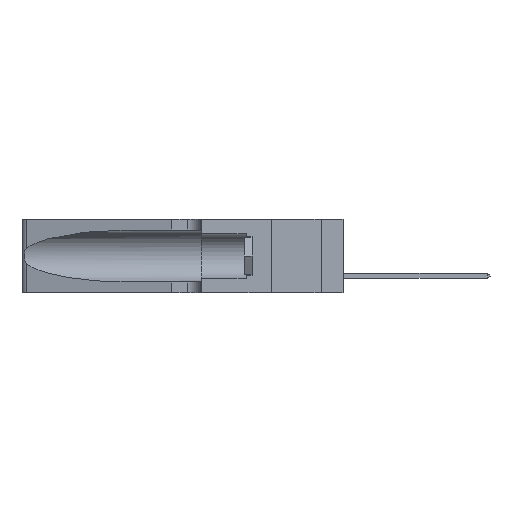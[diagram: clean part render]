
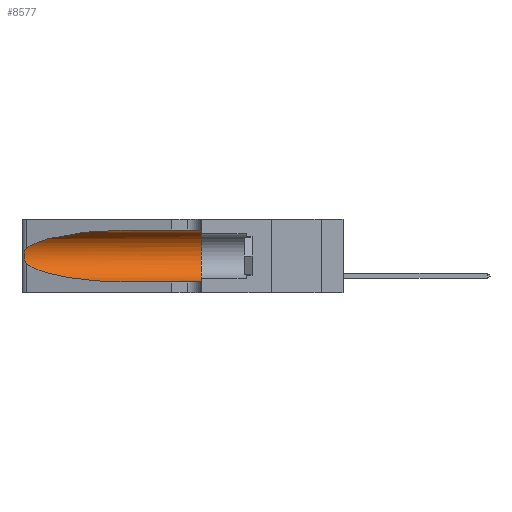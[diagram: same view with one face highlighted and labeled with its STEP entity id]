
A CAD part, left-side view. The second image highlights one B-rep face of the part: STEP entity #8577.
In plain terms, the highlighted cylindrical face has radius 3.308 mm (diameter 6.617 mm), a partial arc.
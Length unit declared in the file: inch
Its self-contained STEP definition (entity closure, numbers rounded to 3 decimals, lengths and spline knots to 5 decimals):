
#87 = CARTESIAN_POINT ( 'NONE',  ( 0.26075, 1.23896, 0.178 ) ) ;
#493 = FACE_OUTER_BOUND ( 'NONE', #5548, .T. ) ;
#574 = CARTESIAN_POINT ( 'NONE',  ( 0.18966, 0.96281, 0.05475 ) ) ;
#796 = CYLINDRICAL_SURFACE ( 'NONE', #13672, 0.13025 ) ;
#1091 = ORIENTED_EDGE ( 'NONE', *, *, #11890, .F. ) ;
#1527 = CARTESIAN_POINT ( 'NONE',  ( 0.25487, 1.22718, 0.14631 ) ) ;
#1621 = VERTEX_POINT ( 'NONE', #1527 ) ;
#1747 = CARTESIAN_POINT ( 'NONE',  ( 0.1305, 0.72297, 0.31525 ) ) ;
#1804 = CARTESIAN_POINT ( 'NONE',  ( 0.25555, 1.22994, 0.2215 ) ) ;
#2199 = DIRECTION ( 'NONE',  ( 0., -1., 0. ) ) ;
#2934 = EDGE_CURVE ( 'NONE', #12074, #1621, #23416, .T. ) ;
#3113 = EDGE_CURVE ( 'NONE', #16441, #12074, #14380, .T. ) ;
#3409 = CARTESIAN_POINT ( 'NONE',  ( 0.1305, 1.61858, 0.185 ) ) ;
#3412 = EDGE_CURVE ( 'NONE', #16441, #20960, #12495, .T. ) ;
#3416 =( BOUNDED_CURVE ( )  B_SPLINE_CURVE ( 3, ( #12030, #18115, #574, #6668 ),
 .UNSPECIFIED., .F., .F. ) 
 B_SPLINE_CURVE_WITH_KNOTS ( ( 4, 4 ),
 ( 3.44316, 4.71239 ),
 .UNSPECIFIED. ) 
 CURVE ( )  GEOMETRIC_REPRESENTATION_ITEM ( )  RATIONAL_B_SPLINE_CURVE ( ( 1., 0.87, 0.87, 1. ) ) 
 REPRESENTATION_ITEM ( '' )  );
#3644 = ORIENTED_EDGE ( 'NONE', *, *, #3113, .T. ) ;
#3799 = CARTESIAN_POINT ( 'NONE',  ( 0.25856, 1.23593, 0.16098 ) ) ;
#3971 = CARTESIAN_POINT ( 'NONE',  ( 0.26018, 1.23835, 0.19895 ) ) ;
#4122 = CARTESIAN_POINT ( 'NONE',  ( 0.25487, 1.22718, 0.22369 ) ) ;
#5021 = CARTESIAN_POINT ( 'NONE',  ( 0.1305, 0.72297, 0.31525 ) ) ;
#5548 = EDGE_LOOP ( 'NONE', ( #3644, #19751, #10902, #11668, #1091, #9495 ) ) ;
#5857 = CARTESIAN_POINT ( 'NONE',  ( 0.25639, 1.23186, 0.15144 ) ) ;
#5880 = CARTESIAN_POINT ( 'NONE',  ( 0.2373, 1.15595, 0.28018 ) ) ;
#6016 = CARTESIAN_POINT ( 'NONE',  ( 0.25487, 1.22718, 0.14631 ) ) ;
#6668 = CARTESIAN_POINT ( 'NONE',  ( 0.1305, 0.72297, 0.05475 ) ) ;
#6704 = DIRECTION ( 'NONE',  ( 0., 0., 1. ) ) ;
#6760 = CIRCLE ( 'NONE', #14863, 0.13025 ) ;
#7250 = CARTESIAN_POINT ( 'NONE',  ( 0.1305, 0.35, 0.31525 ) ) ;
#7749 = CARTESIAN_POINT ( 'NONE',  ( 0.25487, 1.22718, 0.22369 ) ) ;
#8577 = ADVANCED_FACE ( 'NONE', ( #493 ), #796, .F. ) ;
#9495 = ORIENTED_EDGE ( 'NONE', *, *, #3412, .F. ) ;
#9585 = CARTESIAN_POINT ( 'NONE',  ( 0.25639, 1.23184, 0.21858 ) ) ;
#9836 = CARTESIAN_POINT ( 'NONE',  ( 0.25487, 1.22718, 0.22369 ) ) ;
#10902 = ORIENTED_EDGE ( 'NONE', *, *, #11420, .T. ) ;
#11086 = DIRECTION ( 'NONE',  ( 0., 0., -1. ) ) ;
#11402 = LINE ( 'NONE', #13891, #13537 ) ;
#11420 = EDGE_CURVE ( 'NONE', #1621, #20545, #3416, .T. ) ;
#11668 = ORIENTED_EDGE ( 'NONE', *, *, #14832, .T. ) ;
#11890 = EDGE_CURVE ( 'NONE', #20960, #20914, #6760, .T. ) ;
#12030 = CARTESIAN_POINT ( 'NONE',  ( 0.25487, 1.22718, 0.14631 ) ) ;
#12074 = VERTEX_POINT ( 'NONE', #4122 ) ;
#12495 = LINE ( 'NONE', #22731, #14350 ) ;
#13145 = DIRECTION ( 'NONE',  ( 0., -1., 0. ) ) ;
#13496 = CARTESIAN_POINT ( 'NONE',  ( 0.25787, 1.23484, 0.2124 ) ) ;
#13537 = VECTOR ( 'NONE', #2199, 39.37008 ) ;
#13672 = AXIS2_PLACEMENT_3D ( 'NONE', #3409, #13145, #11086 ) ;
#13891 = CARTESIAN_POINT ( 'NONE',  ( 0.1305, 1.61858, 0.05475 ) ) ;
#14350 = VECTOR ( 'NONE', #24687, 39.37008 ) ;
#14380 =( BOUNDED_CURVE ( )  B_SPLINE_CURVE ( 3, ( #1747, #19445, #5880, #7749 ),
 .UNSPECIFIED., .F., .T. ) 
 B_SPLINE_CURVE_WITH_KNOTS ( ( 4, 4 ),
 ( 1.5708, 2.84003 ),
 .UNSPECIFIED. ) 
 CURVE ( )  GEOMETRIC_REPRESENTATION_ITEM ( )  RATIONAL_B_SPLINE_CURVE ( ( 1., 0.87, 0.87, 1. ) ) 
 REPRESENTATION_ITEM ( '' )  );
#14832 = EDGE_CURVE ( 'NONE', #20545, #20914, #11402, .T. ) ;
#14863 = AXIS2_PLACEMENT_3D ( 'NONE', #23909, #16342, #6704 ) ;
#15469 = CARTESIAN_POINT ( 'NONE',  ( 0.26017, 1.23833, 0.17102 ) ) ;
#16342 = DIRECTION ( 'NONE',  ( 0., 1., 0. ) ) ;
#16441 = VERTEX_POINT ( 'NONE', #5021 ) ;
#17356 = CARTESIAN_POINT ( 'NONE',  ( 0.1305, 0.72297, 0.05475 ) ) ;
#17520 = CARTESIAN_POINT ( 'NONE',  ( 0.25789, 1.23486, 0.15765 ) ) ;
#17687 = CARTESIAN_POINT ( 'NONE',  ( 0.25555, 1.22993, 0.14849 ) ) ;
#18115 = CARTESIAN_POINT ( 'NONE',  ( 0.2373, 1.15595, 0.08982 ) ) ;
#19445 = CARTESIAN_POINT ( 'NONE',  ( 0.18966, 0.96281, 0.31525 ) ) ;
#19751 = ORIENTED_EDGE ( 'NONE', *, *, #2934, .T. ) ;
#20545 = VERTEX_POINT ( 'NONE', #17356 ) ;
#20914 = VERTEX_POINT ( 'NONE', #22753 ) ;
#20960 = VERTEX_POINT ( 'NONE', #7250 ) ;
#21338 = CARTESIAN_POINT ( 'NONE',  ( 0.25854, 1.2359, 0.20912 ) ) ;
#22731 = CARTESIAN_POINT ( 'NONE',  ( 0.1305, 1.61858, 0.31525 ) ) ;
#22753 = CARTESIAN_POINT ( 'NONE',  ( 0.1305, 0.35, 0.05475 ) ) ;
#23416 = B_SPLINE_CURVE_WITH_KNOTS ( 'NONE', 3,
 ( #9836, #1804, #9585, #13496, #21338, #3971, #25250, #87, #15469, #3799, #17520, #5857, #17687, #6016 ),
 .UNSPECIFIED., .F., .F.,
 ( 4, 2, 2, 2, 2, 2, 4 ),
 ( 0., 0.00027, 0.00053, 0.00107, 0.0016, 0.00187, 0.00214 ),
 .UNSPECIFIED. ) ;
#23909 = CARTESIAN_POINT ( 'NONE',  ( 0.1305, 0.35, 0.185 ) ) ;
#24687 = DIRECTION ( 'NONE',  ( 0., -1., 0. ) ) ;
#25250 = CARTESIAN_POINT ( 'NONE',  ( 0.26075, 1.23896, 0.19203 ) ) ;
